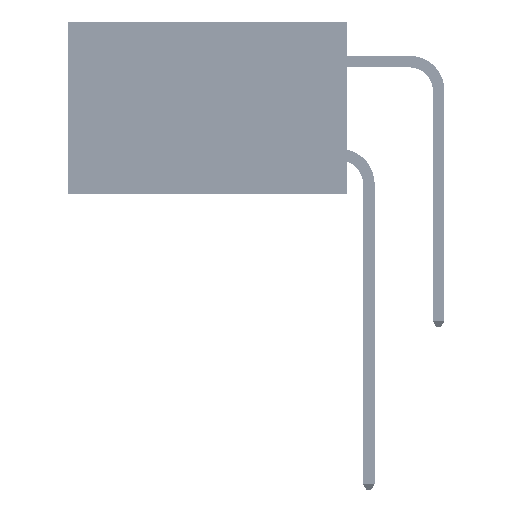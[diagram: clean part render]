
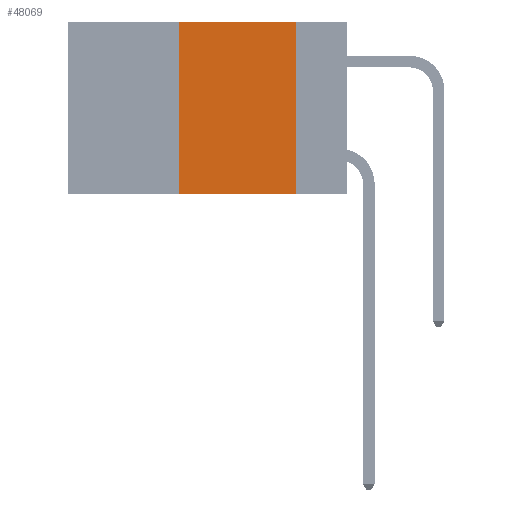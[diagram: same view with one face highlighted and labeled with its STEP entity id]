
A CAD part, left-side view. The second image highlights one B-rep face of the part: STEP entity #48069.
In plain terms, the highlighted planar face has unit normal (-1, 0, 0).
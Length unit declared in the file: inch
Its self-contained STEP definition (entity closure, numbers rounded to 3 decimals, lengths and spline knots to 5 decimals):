
#3239 = FACE_OUTER_BOUND ( 'NONE', #46781, .T. ) ;
#4057 = DIRECTION ( 'NONE',  ( 0., -1., 0. ) ) ;
#4106 = DIRECTION ( 'NONE',  ( 1., 0., 0. ) ) ;
#9606 = CARTESIAN_POINT ( 'NONE',  ( 0., 0.11, 0. ) ) ;
#10615 = EDGE_CURVE ( 'NONE', #34676, #44714, #37528, .T. ) ;
#12021 = ORIENTED_EDGE ( 'NONE', *, *, #10615, .T. ) ;
#12825 = DIRECTION ( 'NONE',  ( 0., -1., 0. ) ) ;
#16587 = CARTESIAN_POINT ( 'NONE',  ( 0., 0.6, 0. ) ) ;
#16684 = EDGE_CURVE ( 'NONE', #34676, #32587, #39865, .T. ) ;
#17545 = CARTESIAN_POINT ( 'NONE',  ( 0., 0.11, -0.37 ) ) ;
#18827 = PLANE ( 'NONE',  #30023 ) ;
#19841 = VECTOR ( 'NONE', #35591, 39.37008 ) ;
#21042 = CARTESIAN_POINT ( 'NONE',  ( 0., 0.36, -0.37 ) ) ;
#21966 = ORIENTED_EDGE ( 'NONE', *, *, #32740, .F. ) ;
#26768 = DIRECTION ( 'NONE',  ( 0., 0., -1. ) ) ;
#27589 = LINE ( 'NONE', #16587, #46361 ) ;
#30011 = VERTEX_POINT ( 'NONE', #9606 ) ;
#30023 = AXIS2_PLACEMENT_3D ( 'NONE', #38135, #4106, #26768 ) ;
#31019 = CARTESIAN_POINT ( 'NONE',  ( 0., 0.6, -0.37 ) ) ;
#31107 = VECTOR ( 'NONE', #4057, 39.37008 ) ;
#32131 = CARTESIAN_POINT ( 'NONE',  ( 0., 0.11, 0. ) ) ;
#32587 = VERTEX_POINT ( 'NONE', #35277 ) ;
#32740 = EDGE_CURVE ( 'NONE', #30011, #44714, #42344, .T. ) ;
#34676 = VERTEX_POINT ( 'NONE', #21042 ) ;
#35277 = CARTESIAN_POINT ( 'NONE',  ( 0., 0.36, 0. ) ) ;
#35591 = DIRECTION ( 'NONE',  ( 0., 0., -1. ) ) ;
#37528 = LINE ( 'NONE', #31019, #31107 ) ;
#38135 = CARTESIAN_POINT ( 'NONE',  ( 0., 0.6, 0. ) ) ;
#38922 = EDGE_CURVE ( 'NONE', #32587, #30011, #27589, .T. ) ;
#39865 = LINE ( 'NONE', #40820, #45813 ) ;
#40820 = CARTESIAN_POINT ( 'NONE',  ( 0., 0.36, 0. ) ) ;
#41916 = ORIENTED_EDGE ( 'NONE', *, *, #16684, .F. ) ;
#41938 = ORIENTED_EDGE ( 'NONE', *, *, #38922, .F. ) ;
#42344 = LINE ( 'NONE', #32131, #19841 ) ;
#44663 = DIRECTION ( 'NONE',  ( 0., 0., 1. ) ) ;
#44714 = VERTEX_POINT ( 'NONE', #17545 ) ;
#45813 = VECTOR ( 'NONE', #44663, 39.37008 ) ;
#46361 = VECTOR ( 'NONE', #12825, 39.37008 ) ;
#46781 = EDGE_LOOP ( 'NONE', ( #21966, #41938, #41916, #12021 ) ) ;
#48069 = ADVANCED_FACE ( 'NONE', ( #3239 ), #18827, .F. ) ;
